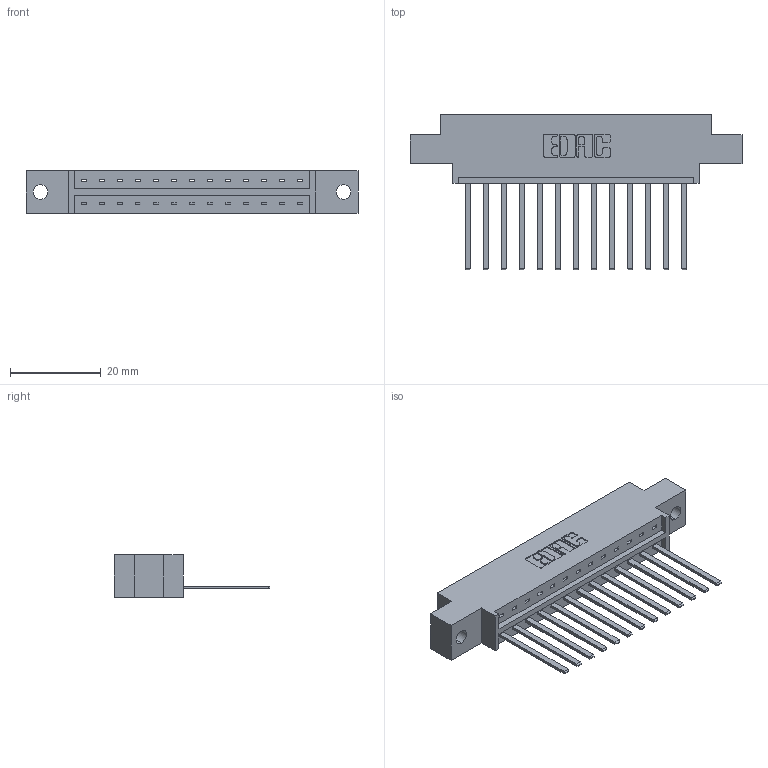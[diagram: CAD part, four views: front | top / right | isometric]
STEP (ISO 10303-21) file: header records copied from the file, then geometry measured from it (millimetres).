
FILE_DESCRIPTION (( 'STEP AP203' ), '1' );
FILE_NAME ('333-013-544-602.STEP', '2018-08-01T01:35:52', ( '' ), ( '' ), 'SwSTEP 2.0', 'SolidWorks 2016', '' );
FILE_SCHEMA (( 'CONFIG_CONTROL_DESIGN' ));
Length unit declared in the file: inch
Products named in the file (3): 333 Part_Offset - .128 Dia; 345-292-001_345-293-144; 333-013-544-602
Assembly tree (14 placements, depth 2):
  333-013-544-602
    333 Part_Offset - .128 Dia
    345-292-001_345-293-144  x13
Bounding box: 73.05 x 34.3 x 9.4 mm (x, y, z)
Volume: 6987.6 mm3; surface area: 7785.9 mm2
Topology: 14 solids, 14 shells, 794 faces, 2377 edges, 1566 vertices
Faces by surface type: plane 568, cylinder 226
Entity records: 11649 total; most frequent: CARTESIAN_POINT 2021, ORIENTED_EDGE 1970, DIRECTION 1759, EDGE_CURVE 985, LINE 861, VECTOR 861, VERTEX_POINT 654, AXIS2_PLACEMENT_3D 449
